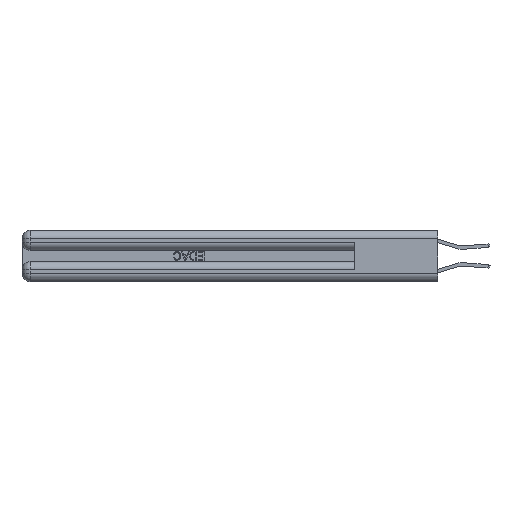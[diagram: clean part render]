
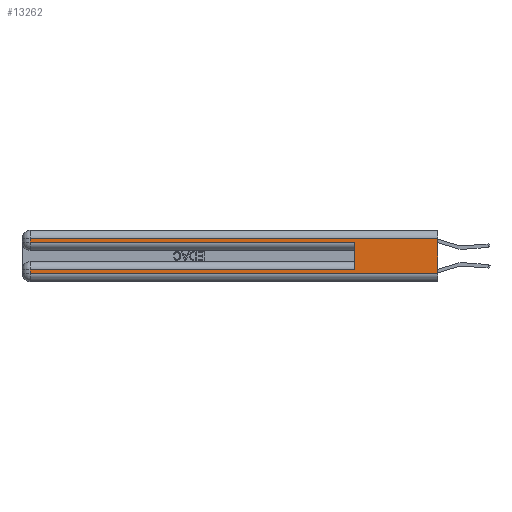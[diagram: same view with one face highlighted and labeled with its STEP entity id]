
A CAD part, left-side view. The second image highlights one B-rep face of the part: STEP entity #13262.
In plain terms, the highlighted planar face has unit normal (-1, 0, 0).
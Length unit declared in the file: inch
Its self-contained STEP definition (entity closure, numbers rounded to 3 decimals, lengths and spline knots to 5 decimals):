
#249 = VERTEX_POINT ( 'NONE', #5331 ) ;
#271 = VECTOR ( 'NONE', #18868, 39.37008 ) ;
#822 = VECTOR ( 'NONE', #4586, 39.37008 ) ;
#825 = CARTESIAN_POINT ( 'NONE',  ( 0., 0.6, 0.145 ) ) ;
#862 = ORIENTED_EDGE ( 'NONE', *, *, #21019, .F. ) ;
#1036 = VERTEX_POINT ( 'NONE', #6882 ) ;
#1060 = LINE ( 'NONE', #7022, #822 ) ;
#2484 = VERTEX_POINT ( 'NONE', #12742 ) ;
#2776 = LINE ( 'NONE', #27663, #19372 ) ;
#2952 = VERTEX_POINT ( 'NONE', #12055 ) ;
#3344 = ORIENTED_EDGE ( 'NONE', *, *, #27334, .T. ) ;
#3604 = DIRECTION ( 'NONE',  ( 0., 1., 0. ) ) ;
#4542 = DIRECTION ( 'NONE',  ( 0., 0., -1. ) ) ;
#4586 = DIRECTION ( 'NONE',  ( 0., -1., 0. ) ) ;
#5331 = CARTESIAN_POINT ( 'NONE',  ( 0., 2.94, 0.31 ) ) ;
#5465 = VECTOR ( 'NONE', #3604, 39.37008 ) ;
#6882 = CARTESIAN_POINT ( 'NONE',  ( 0., 2.94, 0.285 ) ) ;
#6989 = VERTEX_POINT ( 'NONE', #19871 ) ;
#7022 = CARTESIAN_POINT ( 'NONE',  ( 0., 0., 0.285 ) ) ;
#7112 = EDGE_CURVE ( 'NONE', #2952, #12841, #15786, .T. ) ;
#8164 = CARTESIAN_POINT ( 'NONE',  ( 0., 0., 0.085 ) ) ;
#8770 = LINE ( 'NONE', #21794, #271 ) ;
#9055 = ORIENTED_EDGE ( 'NONE', *, *, #7112, .F. ) ;
#9604 = VECTOR ( 'NONE', #31665, 39.37008 ) ;
#10683 = ORIENTED_EDGE ( 'NONE', *, *, #22083, .T. ) ;
#11274 = DIRECTION ( 'NONE',  ( 0., -1., 0. ) ) ;
#12055 = CARTESIAN_POINT ( 'NONE',  ( 0., 0.6, 0.085 ) ) ;
#12395 = CARTESIAN_POINT ( 'NONE',  ( 0., 0., 0.06 ) ) ;
#12742 = CARTESIAN_POINT ( 'NONE',  ( 0., 2.94, 0.085 ) ) ;
#12841 = VERTEX_POINT ( 'NONE', #13619 ) ;
#13171 = VERTEX_POINT ( 'NONE', #27729 ) ;
#13262 = ADVANCED_FACE ( 'NONE', ( #27898 ), #25613, .F. ) ;
#13413 = DIRECTION ( 'NONE',  ( 0., 0., -1. ) ) ;
#13619 = CARTESIAN_POINT ( 'NONE',  ( 0., 0.6, 0.285 ) ) ;
#13646 = ORIENTED_EDGE ( 'NONE', *, *, #15082, .T. ) ;
#15082 = EDGE_CURVE ( 'NONE', #13171, #249, #2776, .T. ) ;
#15786 = LINE ( 'NONE', #825, #29438 ) ;
#15835 = CARTESIAN_POINT ( 'NONE',  ( 0., 0., 0.06 ) ) ;
#16491 = EDGE_CURVE ( 'NONE', #249, #1036, #21781, .T. ) ;
#17877 = VECTOR ( 'NONE', #11274, 39.37008 ) ;
#17991 = CARTESIAN_POINT ( 'NONE',  ( 0., 0., 0.37 ) ) ;
#18084 = DIRECTION ( 'NONE',  ( 0., 1., 0. ) ) ;
#18281 = LINE ( 'NONE', #15835, #17877 ) ;
#18639 = EDGE_LOOP ( 'NONE', ( #862, #13646, #20182, #24010, #9055, #26768, #3344, #10683 ) ) ;
#18868 = DIRECTION ( 'NONE',  ( 0., 0., -1. ) ) ;
#19372 = VECTOR ( 'NONE', #18084, 39.37008 ) ;
#19512 = LINE ( 'NONE', #29721, #26867 ) ;
#19871 = CARTESIAN_POINT ( 'NONE',  ( 0., 2.94, 0.06 ) ) ;
#20182 = ORIENTED_EDGE ( 'NONE', *, *, #16491, .T. ) ;
#21019 = EDGE_CURVE ( 'NONE', #13171, #31131, #19512, .T. ) ;
#21781 = LINE ( 'NONE', #28752, #9604 ) ;
#21794 = CARTESIAN_POINT ( 'NONE',  ( 0., 2.94, 0.37 ) ) ;
#22083 = EDGE_CURVE ( 'NONE', #6989, #31131, #18281, .T. ) ;
#24010 = ORIENTED_EDGE ( 'NONE', *, *, #28347, .T. ) ;
#25146 = DIRECTION ( 'NONE',  ( 1., 0., 0. ) ) ;
#25549 = EDGE_CURVE ( 'NONE', #2952, #2484, #30272, .T. ) ;
#25613 = PLANE ( 'NONE',  #29656 ) ;
#26768 = ORIENTED_EDGE ( 'NONE', *, *, #25549, .T. ) ;
#26867 = VECTOR ( 'NONE', #4542, 39.37008 ) ;
#27334 = EDGE_CURVE ( 'NONE', #2484, #6989, #8770, .T. ) ;
#27663 = CARTESIAN_POINT ( 'NONE',  ( 0., 0., 0.31 ) ) ;
#27729 = CARTESIAN_POINT ( 'NONE',  ( 0., 0., 0.31 ) ) ;
#27898 = FACE_OUTER_BOUND ( 'NONE', #18639, .T. ) ;
#28295 = DIRECTION ( 'NONE',  ( 0., 0., 1. ) ) ;
#28347 = EDGE_CURVE ( 'NONE', #1036, #12841, #1060, .T. ) ;
#28752 = CARTESIAN_POINT ( 'NONE',  ( 0., 2.94, 0.37 ) ) ;
#29438 = VECTOR ( 'NONE', #28295, 39.37008 ) ;
#29656 = AXIS2_PLACEMENT_3D ( 'NONE', #17991, #25146, #13413 ) ;
#29721 = CARTESIAN_POINT ( 'NONE',  ( 0., 0., 0.37 ) ) ;
#30272 = LINE ( 'NONE', #8164, #5465 ) ;
#31131 = VERTEX_POINT ( 'NONE', #12395 ) ;
#31665 = DIRECTION ( 'NONE',  ( 0., 0., -1. ) ) ;
